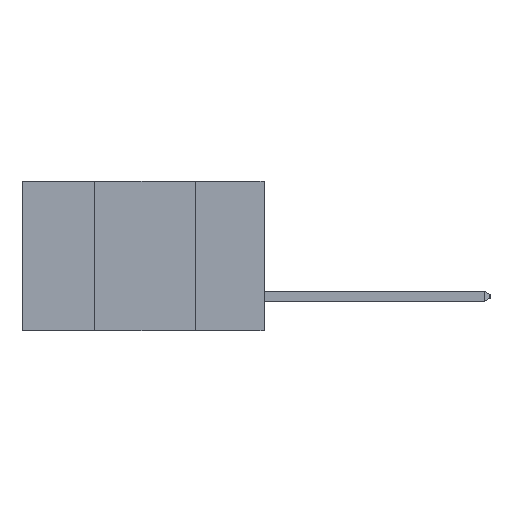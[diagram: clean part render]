
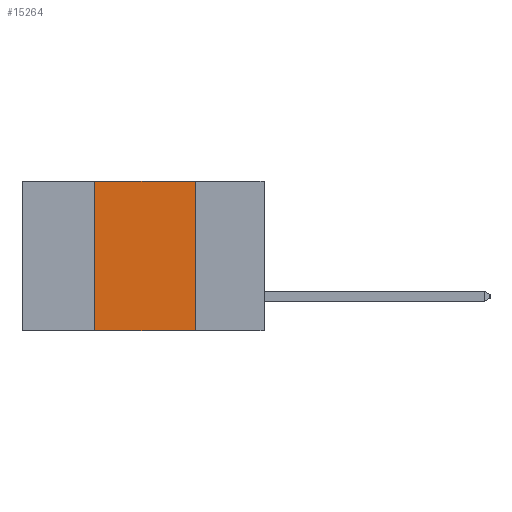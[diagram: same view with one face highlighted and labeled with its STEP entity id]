
A CAD part, left-side view. The second image highlights one B-rep face of the part: STEP entity #15264.
In plain terms, the highlighted planar face has unit normal (-1, 0, 0).
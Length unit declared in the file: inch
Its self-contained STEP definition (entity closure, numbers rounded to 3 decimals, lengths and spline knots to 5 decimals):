
#55 = VERTEX_POINT ( 'NONE', #16638 ) ;
#267 = LINE ( 'NONE', #16029, #14597 ) ;
#474 = ORIENTED_EDGE ( 'NONE', *, *, #6213, .F. ) ;
#570 = FACE_OUTER_BOUND ( 'NONE', #15697, .T. ) ;
#848 = LINE ( 'NONE', #3648, #11537 ) ;
#1799 = LINE ( 'NONE', #5574, #2238 ) ;
#2017 = DIRECTION ( 'NONE',  ( 0., 0., -1. ) ) ;
#2238 = VECTOR ( 'NONE', #5512, 39.37008 ) ;
#2375 = CARTESIAN_POINT ( 'NONE',  ( 0., 0.42, -0.37 ) ) ;
#2974 = VECTOR ( 'NONE', #10078, 39.37008 ) ;
#3025 = CARTESIAN_POINT ( 'NONE',  ( 0., 0.17, -0.37 ) ) ;
#3648 = CARTESIAN_POINT ( 'NONE',  ( 0., 0.6, -0.37 ) ) ;
#5512 = DIRECTION ( 'NONE',  ( 0., 0., 1. ) ) ;
#5574 = CARTESIAN_POINT ( 'NONE',  ( 0., 0.42, -0.37 ) ) ;
#5613 = CARTESIAN_POINT ( 'NONE',  ( 0., 0.17, -0.37 ) ) ;
#6213 = EDGE_CURVE ( 'NONE', #11365, #12141, #10841, .T. ) ;
#6450 = DIRECTION ( 'NONE',  ( 0., -1., 0. ) ) ;
#7273 = ORIENTED_EDGE ( 'NONE', *, *, #13373, .F. ) ;
#7603 = PLANE ( 'NONE',  #14939 ) ;
#8333 = EDGE_CURVE ( 'NONE', #55, #11365, #267, .T. ) ;
#9018 = CARTESIAN_POINT ( 'NONE',  ( 0., 0.6, 0. ) ) ;
#10078 = DIRECTION ( 'NONE',  ( 0., 0., -1. ) ) ;
#10416 = DIRECTION ( 'NONE',  ( 1., 0., 0. ) ) ;
#10841 = LINE ( 'NONE', #3025, #2974 ) ;
#11365 = VERTEX_POINT ( 'NONE', #14339 ) ;
#11537 = VECTOR ( 'NONE', #17462, 39.37008 ) ;
#11818 = ORIENTED_EDGE ( 'NONE', *, *, #13847, .T. ) ;
#12141 = VERTEX_POINT ( 'NONE', #5613 ) ;
#13373 = EDGE_CURVE ( 'NONE', #15458, #55, #1799, .T. ) ;
#13727 = ORIENTED_EDGE ( 'NONE', *, *, #8333, .F. ) ;
#13847 = EDGE_CURVE ( 'NONE', #15458, #12141, #848, .T. ) ;
#14339 = CARTESIAN_POINT ( 'NONE',  ( 0., 0.17, 0. ) ) ;
#14597 = VECTOR ( 'NONE', #6450, 39.37008 ) ;
#14939 = AXIS2_PLACEMENT_3D ( 'NONE', #9018, #10416, #2017 ) ;
#15264 = ADVANCED_FACE ( 'NONE', ( #570 ), #7603, .F. ) ;
#15458 = VERTEX_POINT ( 'NONE', #2375 ) ;
#15697 = EDGE_LOOP ( 'NONE', ( #474, #13727, #7273, #11818 ) ) ;
#16029 = CARTESIAN_POINT ( 'NONE',  ( 0., 0.6, 0. ) ) ;
#16638 = CARTESIAN_POINT ( 'NONE',  ( 0., 0.42, 0. ) ) ;
#17462 = DIRECTION ( 'NONE',  ( 0., -1., 0. ) ) ;
